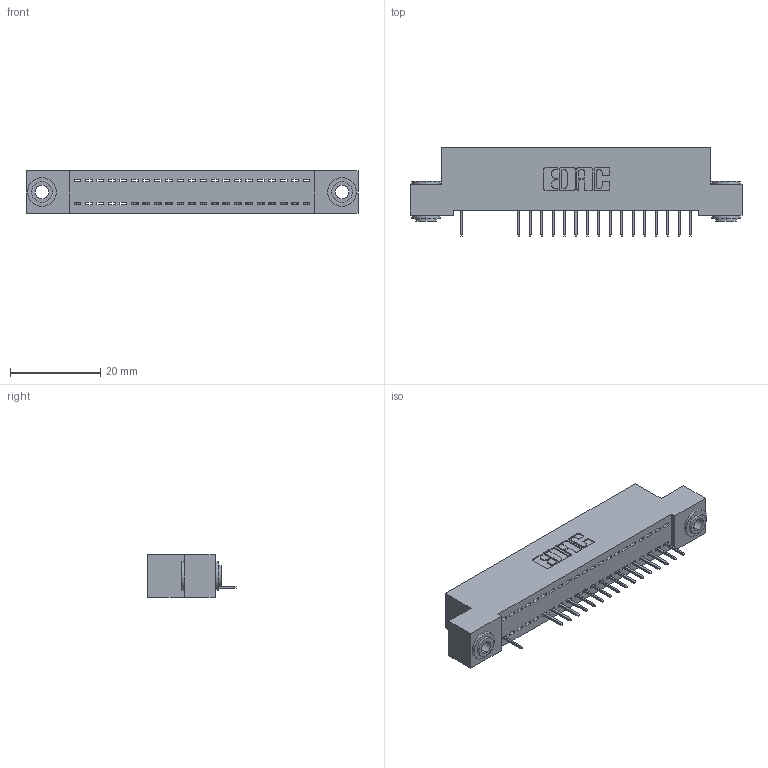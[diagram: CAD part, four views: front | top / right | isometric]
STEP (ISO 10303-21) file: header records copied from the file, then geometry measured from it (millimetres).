
FILE_DESCRIPTION (( 'STEP AP203' ), '1' );
FILE_NAME ('392-021-524-103.STEP', '2018-08-15T07:47:22', ( '' ), ( '' ), 'SwSTEP 2.0', 'SolidWorks 2016', '' );
FILE_SCHEMA (( 'CONFIG_CONTROL_DESIGN' ));
Length unit declared in the file: inch
Products named in the file (4): 342 Part_.156 TH; 345-292-001_345-293-124; 342-250-002_345-250-002-102; 392-021-524-103
Assembly tree (20 placements, depth 2):
  392-021-524-103
    342 Part_.156 TH
    345-292-001_345-293-124  x17
    342-250-002_345-250-002-102  x2
Bounding box: 73.66 x 19.69 x 9.4 mm (x, y, z)
Volume: 6291.1 mm3; surface area: 8626.6 mm2
Topology: 20 solids, 20 shells, 1250 faces, 3603 edges, 2330 vertices
Faces by surface type: plane 940, cylinder 302, cone 8
Entity records: 16018 total; most frequent: CARTESIAN_POINT 2760, ORIENTED_EDGE 2714, DIRECTION 2401, EDGE_CURVE 1357, VECTOR 1209, LINE 1209, VERTEX_POINT 898, AXIS2_PLACEMENT_3D 596
